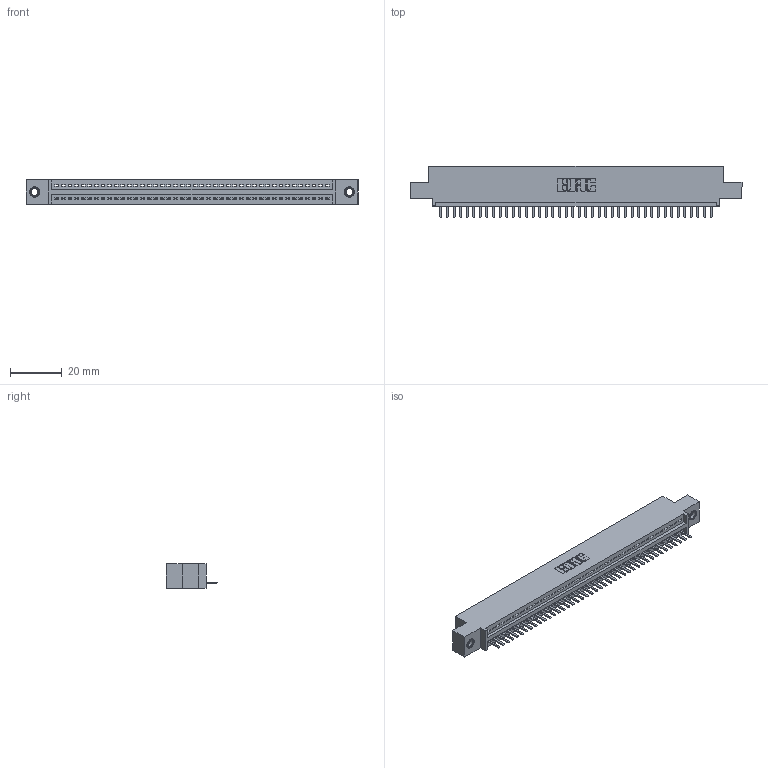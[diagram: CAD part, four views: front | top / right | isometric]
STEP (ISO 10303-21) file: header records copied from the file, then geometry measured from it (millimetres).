
FILE_DESCRIPTION (( 'STEP AP203' ), '1' );
FILE_NAME ('395-042-520-407.STEP', '2018-11-15T07:23:52', ( '' ), ( '' ), 'SwSTEP 2.0', 'SolidWorks 2016', '' );
FILE_SCHEMA (( 'CONFIG_CONTROL_DESIGN' ));
Length unit declared in the file: inch
Products named in the file (4): 345-250-001_345-250-005-103; 345 Part_0.110 Offset - 0.156 Dia-TI; 395-042-520-407; 345-292-001_345-293-120
Assembly tree (45 placements, depth 2):
  395-042-520-407
    345 Part_0.110 Offset - 0.156 Dia-TI
    345-292-001_345-293-120  x42
    345-250-001_345-250-005-103  x2
Bounding box: 127.89 x 19.68 x 9.4 mm (x, y, z)
Volume: 11939.3 mm3; surface area: 15585.5 mm2
Topology: 45 solids, 45 shells, 2794 faces, 8217 edges, 5358 vertices
Faces by surface type: plane 1880, cylinder 898, cone 12, torus 4
Entity records: 33042 total; most frequent: CARTESIAN_POINT 5717, ORIENTED_EDGE 5674, DIRECTION 5007, EDGE_CURVE 2837, LINE 2513, VECTOR 2513, VERTEX_POINT 1884, AXIS2_PLACEMENT_3D 1247
